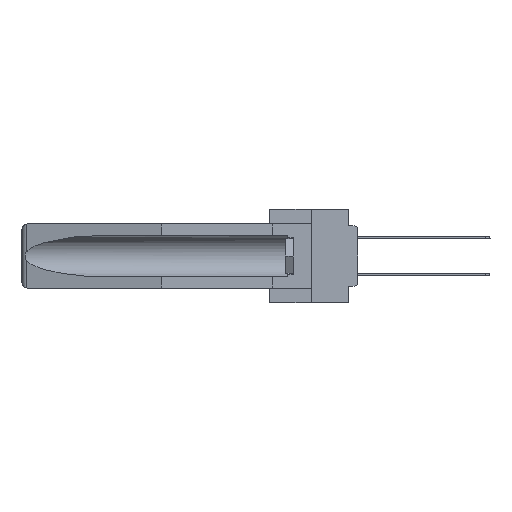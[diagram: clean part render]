
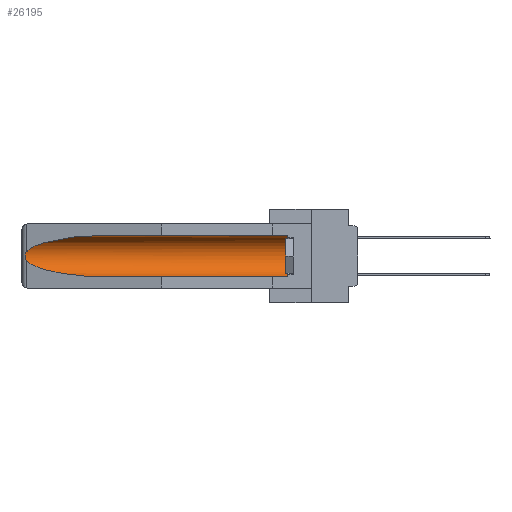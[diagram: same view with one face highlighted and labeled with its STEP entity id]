
A CAD part, left-side view. The second image highlights one B-rep face of the part: STEP entity #26195.
In plain terms, the highlighted cylindrical face has radius 2.857 mm (diameter 5.715 mm), a partial arc.
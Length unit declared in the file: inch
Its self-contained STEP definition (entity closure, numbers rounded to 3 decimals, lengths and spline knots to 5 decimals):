
#2099 = CARTESIAN_POINT ( 'NONE',  ( 0.26537, 1.52718, -0.19328 ) ) ;
#2283 = CARTESIAN_POINT ( 'NONE',  ( 0.155, 0.126, -0.059 ) ) ;
#2689 = CARTESIAN_POINT ( 'NONE',  ( 0.155, 1.07973, -0.284 ) ) ;
#2806 = CARTESIAN_POINT ( 'NONE',  ( 0.155, 1.07973, -0.284 ) ) ;
#3120 = DIRECTION ( 'NONE',  ( 0., 1., 0. ) ) ;
#3509 = EDGE_LOOP ( 'NONE', ( #16142, #26314, #35049, #5370, #13659, #25566 ) ) ;
#4062 =( BOUNDED_CURVE ( )  B_SPLINE_CURVE ( 3, ( #2099, #12970, #34869, #2806 ),
 .UNSPECIFIED., .F., .T. ) 
 B_SPLINE_CURVE_WITH_KNOTS ( ( 4, 4 ),
 ( 0.1948, 1.5708 ),
 .UNSPECIFIED. ) 
 CURVE ( )  GEOMETRIC_REPRESENTATION_ITEM ( )  RATIONAL_B_SPLINE_CURVE ( ( 1., 0.848, 0.848, 1. ) ) 
 REPRESENTATION_ITEM ( '' )  );
#4270 =( BOUNDED_CURVE ( )  B_SPLINE_CURVE ( 3, ( #16664, #11504, #18984, #13625 ),
 .UNSPECIFIED., .F., .T. ) 
 B_SPLINE_CURVE_WITH_KNOTS ( ( 4, 4 ),
 ( 4.71239, 6.08839 ),
 .UNSPECIFIED. ) 
 CURVE ( )  GEOMETRIC_REPRESENTATION_ITEM ( )  RATIONAL_B_SPLINE_CURVE ( ( 1., 0.848, 0.848, 1. ) ) 
 REPRESENTATION_ITEM ( '' )  );
#5218 = DIRECTION ( 'NONE',  ( 0., 1., 0. ) ) ;
#5297 = CARTESIAN_POINT ( 'NONE',  ( 0.26537, 1.52718, -0.19328 ) ) ;
#5370 = ORIENTED_EDGE ( 'NONE', *, *, #26879, .F. ) ;
#5597 = DIRECTION ( 'NONE',  ( 0., 0., 1. ) ) ;
#5890 = LINE ( 'NONE', #13894, #9778 ) ;
#6082 = CIRCLE ( 'NONE', #28828, 0.1125 ) ;
#7258 = EDGE_CURVE ( 'NONE', #30107, #12188, #4062, .T. ) ;
#8079 = CARTESIAN_POINT ( 'NONE',  ( 0.155, -0.30754, -0.1715 ) ) ;
#8222 = CARTESIAN_POINT ( 'NONE',  ( 0.26654, 1.53092, -0.15636 ) ) ;
#9778 = VECTOR ( 'NONE', #16755, 39.37008 ) ;
#10897 = CARTESIAN_POINT ( 'NONE',  ( 0.26597, 1.5296, -0.19026 ) ) ;
#10948 = DIRECTION ( 'NONE',  ( 0., -1., 0. ) ) ;
#11504 = CARTESIAN_POINT ( 'NONE',  ( 0.21114, 1.30732, -0.059 ) ) ;
#12147 = EDGE_CURVE ( 'NONE', #15629, #30107, #22364, .T. ) ;
#12188 = VERTEX_POINT ( 'NONE', #2689 ) ;
#12970 = CARTESIAN_POINT ( 'NONE',  ( 0.25451, 1.48313, -0.24835 ) ) ;
#13172 = VERTEX_POINT ( 'NONE', #30792 ) ;
#13184 = CARTESIAN_POINT ( 'NONE',  ( 0.26537, 1.52718, -0.14972 ) ) ;
#13206 = CARTESIAN_POINT ( 'NONE',  ( 0.2675, 1.53308, -0.16763 ) ) ;
#13625 = CARTESIAN_POINT ( 'NONE',  ( 0.26537, 1.52718, -0.14972 ) ) ;
#13659 = ORIENTED_EDGE ( 'NONE', *, *, #34574, .T. ) ;
#13894 = CARTESIAN_POINT ( 'NONE',  ( 0.155, -0.30754, -0.284 ) ) ;
#13908 = CARTESIAN_POINT ( 'NONE',  ( 0.26597, 1.52961, -0.15275 ) ) ;
#15629 = VERTEX_POINT ( 'NONE', #13184 ) ;
#16055 = CARTESIAN_POINT ( 'NONE',  ( 0.26537, 1.52718, -0.14972 ) ) ;
#16142 = ORIENTED_EDGE ( 'NONE', *, *, #30722, .T. ) ;
#16409 = CARTESIAN_POINT ( 'NONE',  ( 0.2673, 1.5327, -0.16383 ) ) ;
#16664 = CARTESIAN_POINT ( 'NONE',  ( 0.155, 1.07973, -0.059 ) ) ;
#16755 = DIRECTION ( 'NONE',  ( 0., 1., 0. ) ) ;
#18965 = CARTESIAN_POINT ( 'NONE',  ( 0.155, 0.126, -0.1715 ) ) ;
#18984 = CARTESIAN_POINT ( 'NONE',  ( 0.25451, 1.48313, -0.09465 ) ) ;
#19121 = FACE_OUTER_BOUND ( 'NONE', #3509, .T. ) ;
#20127 = VERTEX_POINT ( 'NONE', #33349 ) ;
#22364 = B_SPLINE_CURVE_WITH_KNOTS ( 'NONE', 3,
 ( #16055, #13908, #8222, #16409, #13206, #24079, #26934, #24608, #10897, #24257 ),
 .UNSPECIFIED., .F., .F.,
 ( 4, 2, 2, 2, 4 ),
 ( 0., 0.00029, 0.00058, 0.00087, 0.00117 ),
 .UNSPECIFIED. ) ;
#22780 = EDGE_CURVE ( 'NONE', #28473, #20127, #27355, .T. ) ;
#23371 = AXIS2_PLACEMENT_3D ( 'NONE', #8079, #5218, #29293 ) ;
#24079 = CARTESIAN_POINT ( 'NONE',  ( 0.2675, 1.53308, -0.17534 ) ) ;
#24257 = CARTESIAN_POINT ( 'NONE',  ( 0.26537, 1.52718, -0.19328 ) ) ;
#24608 = CARTESIAN_POINT ( 'NONE',  ( 0.26655, 1.53094, -0.18657 ) ) ;
#25566 = ORIENTED_EDGE ( 'NONE', *, *, #22780, .T. ) ;
#26195 = ADVANCED_FACE ( 'NONE', ( #19121 ), #32656, .F. ) ;
#26314 = ORIENTED_EDGE ( 'NONE', *, *, #12147, .T. ) ;
#26879 = EDGE_CURVE ( 'NONE', #13172, #12188, #5890, .T. ) ;
#26934 = CARTESIAN_POINT ( 'NONE',  ( 0.2673, 1.53269, -0.17917 ) ) ;
#27355 = LINE ( 'NONE', #29864, #28439 ) ;
#28439 = VECTOR ( 'NONE', #3120, 39.37008 ) ;
#28473 = VERTEX_POINT ( 'NONE', #2283 ) ;
#28828 = AXIS2_PLACEMENT_3D ( 'NONE', #18965, #10948, #5597 ) ;
#29293 = DIRECTION ( 'NONE',  ( 0., 0., 1. ) ) ;
#29864 = CARTESIAN_POINT ( 'NONE',  ( 0.155, -0.30754, -0.059 ) ) ;
#30107 = VERTEX_POINT ( 'NONE', #5297 ) ;
#30722 = EDGE_CURVE ( 'NONE', #20127, #15629, #4270, .T. ) ;
#30792 = CARTESIAN_POINT ( 'NONE',  ( 0.155, 0.126, -0.284 ) ) ;
#32656 = CYLINDRICAL_SURFACE ( 'NONE', #23371, 0.1125 ) ;
#33349 = CARTESIAN_POINT ( 'NONE',  ( 0.155, 1.07973, -0.059 ) ) ;
#34574 = EDGE_CURVE ( 'NONE', #13172, #28473, #6082, .T. ) ;
#34869 = CARTESIAN_POINT ( 'NONE',  ( 0.21114, 1.30732, -0.284 ) ) ;
#35049 = ORIENTED_EDGE ( 'NONE', *, *, #7258, .T. ) ;
